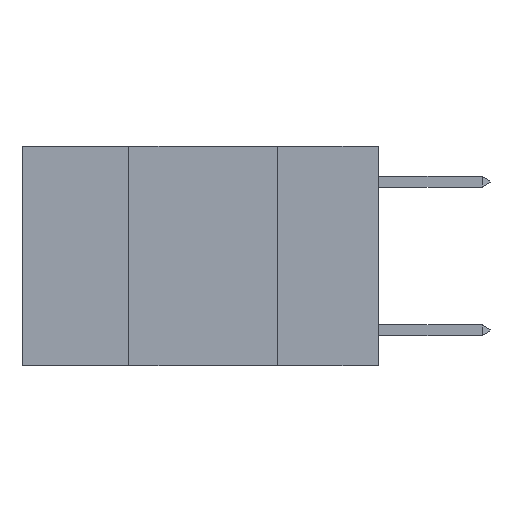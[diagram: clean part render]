
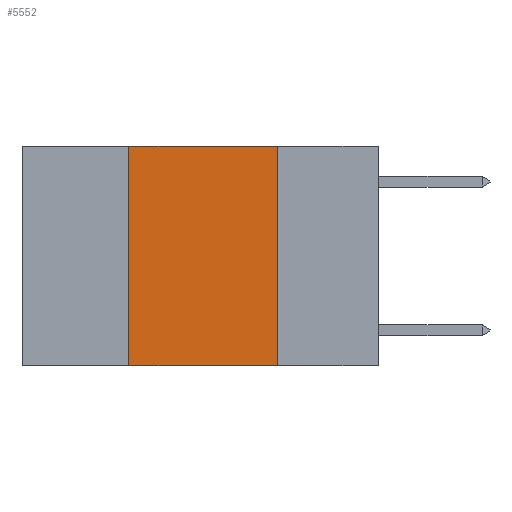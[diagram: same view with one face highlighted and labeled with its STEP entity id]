
A CAD part, left-side view. The second image highlights one B-rep face of the part: STEP entity #5552.
In plain terms, the highlighted planar face has unit normal (-1, 0, 0).
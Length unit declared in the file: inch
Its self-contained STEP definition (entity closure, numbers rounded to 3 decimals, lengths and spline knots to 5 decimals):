
#11 = CARTESIAN_POINT ( 'NONE',  ( 0., 0.42, -0.37 ) ) ;
#1189 = CARTESIAN_POINT ( 'NONE',  ( 0., 0.6, 0. ) ) ;
#1321 = EDGE_CURVE ( 'NONE', #8518, #12824, #3221, .T. ) ;
#1432 = FACE_OUTER_BOUND ( 'NONE', #8143, .T. ) ;
#1480 = VECTOR ( 'NONE', #5422, 39.37008 ) ;
#2180 = DIRECTION ( 'NONE',  ( 0., -1., 0. ) ) ;
#2692 = LINE ( 'NONE', #13466, #1480 ) ;
#3022 = VERTEX_POINT ( 'NONE', #13536 ) ;
#3221 = LINE ( 'NONE', #5042, #3468 ) ;
#3468 = VECTOR ( 'NONE', #7849, 39.37008 ) ;
#4758 = LINE ( 'NONE', #10157, #15055 ) ;
#5042 = CARTESIAN_POINT ( 'NONE',  ( 0., 0.17, 0. ) ) ;
#5422 = DIRECTION ( 'NONE',  ( 0., -1., 0. ) ) ;
#5552 = ADVANCED_FACE ( 'NONE', ( #1432 ), #16279, .F. ) ;
#6207 = ORIENTED_EDGE ( 'NONE', *, *, #12185, .F. ) ;
#7015 = VERTEX_POINT ( 'NONE', #11 ) ;
#7849 = DIRECTION ( 'NONE',  ( 0., 0., -1. ) ) ;
#8043 = LINE ( 'NONE', #12115, #8757 ) ;
#8143 = EDGE_LOOP ( 'NONE', ( #10142, #15199, #6207, #16425 ) ) ;
#8518 = VERTEX_POINT ( 'NONE', #16574 ) ;
#8757 = VECTOR ( 'NONE', #16268, 39.37008 ) ;
#10142 = ORIENTED_EDGE ( 'NONE', *, *, #1321, .F. ) ;
#10157 = CARTESIAN_POINT ( 'NONE',  ( 0., 0.6, -0.37 ) ) ;
#12050 = DIRECTION ( 'NONE',  ( 1., 0., 0. ) ) ;
#12115 = CARTESIAN_POINT ( 'NONE',  ( 0., 0.42, 0. ) ) ;
#12185 = EDGE_CURVE ( 'NONE', #7015, #3022, #8043, .T. ) ;
#12805 = EDGE_CURVE ( 'NONE', #7015, #12824, #4758, .T. ) ;
#12824 = VERTEX_POINT ( 'NONE', #13146 ) ;
#13146 = CARTESIAN_POINT ( 'NONE',  ( 0., 0.17, -0.37 ) ) ;
#13445 = AXIS2_PLACEMENT_3D ( 'NONE', #1189, #12050, #14850 ) ;
#13466 = CARTESIAN_POINT ( 'NONE',  ( 0., 0.6, 0. ) ) ;
#13536 = CARTESIAN_POINT ( 'NONE',  ( 0., 0.42, 0. ) ) ;
#14850 = DIRECTION ( 'NONE',  ( 0., 0., -1. ) ) ;
#15055 = VECTOR ( 'NONE', #2180, 39.37008 ) ;
#15199 = ORIENTED_EDGE ( 'NONE', *, *, #16810, .F. ) ;
#16268 = DIRECTION ( 'NONE',  ( 0., 0., 1. ) ) ;
#16279 = PLANE ( 'NONE',  #13445 ) ;
#16425 = ORIENTED_EDGE ( 'NONE', *, *, #12805, .T. ) ;
#16574 = CARTESIAN_POINT ( 'NONE',  ( 0., 0.17, 0. ) ) ;
#16810 = EDGE_CURVE ( 'NONE', #3022, #8518, #2692, .T. ) ;
